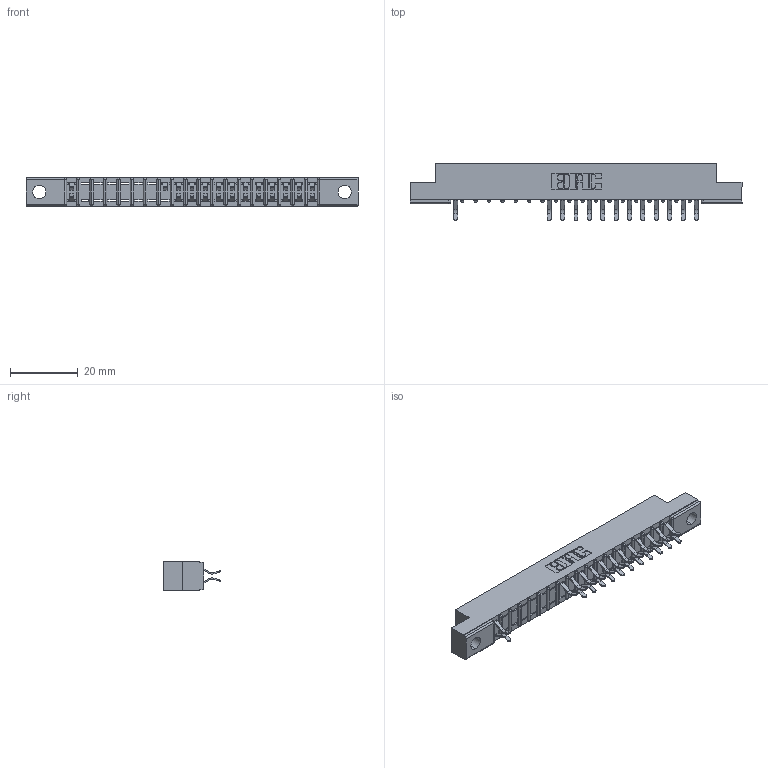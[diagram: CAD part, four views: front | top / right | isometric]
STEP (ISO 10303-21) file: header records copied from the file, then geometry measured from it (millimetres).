
FILE_DESCRIPTION (( 'STEP AP203' ), '1' );
FILE_NAME ('307-038-556-204.STEP', '2018-08-05T12:00:02', ( '' ), ( '' ), 'SwSTEP 2.0', 'SolidWorks 2016', '' );
FILE_SCHEMA (( 'CONFIG_CONTROL_DESIGN' ));
Length unit declared in the file: inch
Products named in the file (3): 307 Part_.156 Dia Mounting Holes; 307-290-001_556; 307-038-556-204
Assembly tree (26 placements, depth 2):
  307-038-556-204
    307 Part_.156 Dia Mounting Holes
    307-290-001_556  x25
Bounding box: 98.3 x 16.97 x 8.71 mm (x, y, z)
Volume: 6151.3 mm3; surface area: 9577.7 mm2
Topology: 26 solids, 26 shells, 1532 faces, 4325 edges, 2794 vertices
Faces by surface type: plane 987, cylinder 505, sphere 40
Entity records: 19838 total; most frequent: CARTESIAN_POINT 3312, ORIENTED_EDGE 3290, DIRECTION 3233, EDGE_CURVE 1645, VECTOR 1259, LINE 1259, VERTEX_POINT 1066, AXIS2_PLACEMENT_3D 987
